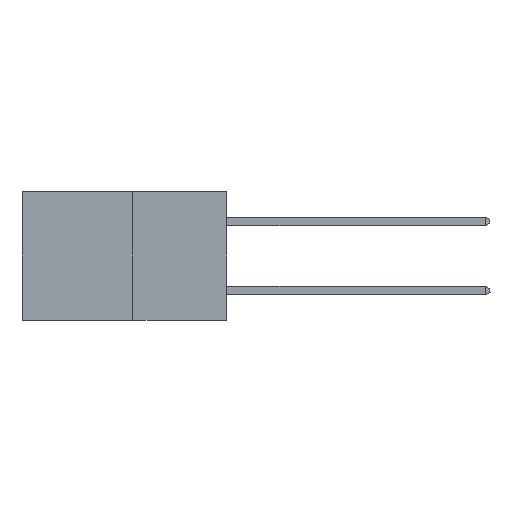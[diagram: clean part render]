
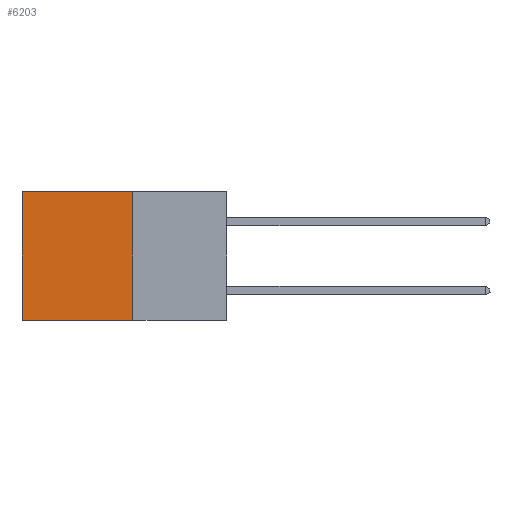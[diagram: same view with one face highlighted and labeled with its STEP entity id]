
A CAD part, left-side view. The second image highlights one B-rep face of the part: STEP entity #6203.
In plain terms, the highlighted planar face has unit normal (-1, 0, 0).
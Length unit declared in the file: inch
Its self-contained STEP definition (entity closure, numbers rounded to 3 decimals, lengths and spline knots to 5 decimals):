
#10 = CARTESIAN_POINT ( 'NONE',  ( 0.277, 0.27, 0. ) ) ;
#27 = LINE ( 'NONE', #8151, #8415 ) ;
#318 = VECTOR ( 'NONE', #7733, 39.37008 ) ;
#497 = EDGE_CURVE ( 'NONE', #8746, #6911, #27, .T. ) ;
#541 = DIRECTION ( 'NONE',  ( 0., 1., 0. ) ) ;
#1948 = EDGE_CURVE ( 'NONE', #5687, #6911, #6943, .T. ) ;
#2467 = LINE ( 'NONE', #6981, #318 ) ;
#2781 = VECTOR ( 'NONE', #4909, 39.37008 ) ;
#2807 = DIRECTION ( 'NONE',  ( 0., 0., -1. ) ) ;
#2831 = ORIENTED_EDGE ( 'NONE', *, *, #7899, .T. ) ;
#3014 = AXIS2_PLACEMENT_3D ( 'NONE', #6715, #7468, #2807 ) ;
#3155 = CARTESIAN_POINT ( 'NONE',  ( 0.277, 0.59, 0. ) ) ;
#3427 = CARTESIAN_POINT ( 'NONE',  ( 0.277, 0.59, -0.37 ) ) ;
#4238 = ORIENTED_EDGE ( 'NONE', *, *, #497, .F. ) ;
#4739 = CARTESIAN_POINT ( 'NONE',  ( 0.277, 0.59, -0.37 ) ) ;
#4909 = DIRECTION ( 'NONE',  ( 0., 0., -1. ) ) ;
#5200 = PLANE ( 'NONE',  #3014 ) ;
#5316 = VERTEX_POINT ( 'NONE', #10 ) ;
#5631 = EDGE_CURVE ( 'NONE', #5316, #8746, #2467, .T. ) ;
#5687 = VERTEX_POINT ( 'NONE', #3155 ) ;
#5731 = FACE_OUTER_BOUND ( 'NONE', #9568, .T. ) ;
#5878 = CARTESIAN_POINT ( 'NONE',  ( 0.277, 0.27, 0. ) ) ;
#5939 = ORIENTED_EDGE ( 'NONE', *, *, #5631, .F. ) ;
#6203 = ADVANCED_FACE ( 'NONE', ( #5731 ), #5200, .F. ) ;
#6512 = ORIENTED_EDGE ( 'NONE', *, *, #1948, .T. ) ;
#6634 = DIRECTION ( 'NONE',  ( 0., 1., 0. ) ) ;
#6715 = CARTESIAN_POINT ( 'NONE',  ( 0.277, 0.27, -0.37 ) ) ;
#6716 = CARTESIAN_POINT ( 'NONE',  ( 0.277, 0.27, -0.37 ) ) ;
#6911 = VERTEX_POINT ( 'NONE', #3427 ) ;
#6943 = LINE ( 'NONE', #4739, #2781 ) ;
#6981 = CARTESIAN_POINT ( 'NONE',  ( 0.277, 0.27, -0.37 ) ) ;
#7468 = DIRECTION ( 'NONE',  ( 1., 0., 0. ) ) ;
#7733 = DIRECTION ( 'NONE',  ( 0., 0., -1. ) ) ;
#7899 = EDGE_CURVE ( 'NONE', #5316, #5687, #8868, .T. ) ;
#8151 = CARTESIAN_POINT ( 'NONE',  ( 0.277, 0.27, -0.37 ) ) ;
#8415 = VECTOR ( 'NONE', #541, 39.37008 ) ;
#8632 = VECTOR ( 'NONE', #6634, 39.37008 ) ;
#8746 = VERTEX_POINT ( 'NONE', #6716 ) ;
#8868 = LINE ( 'NONE', #5878, #8632 ) ;
#9568 = EDGE_LOOP ( 'NONE', ( #6512, #4238, #5939, #2831 ) ) ;
